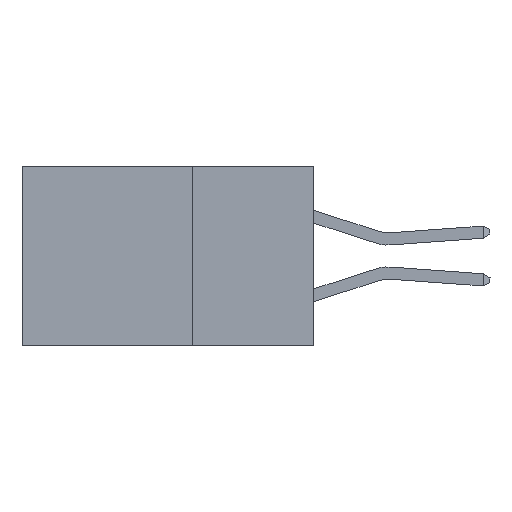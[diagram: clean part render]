
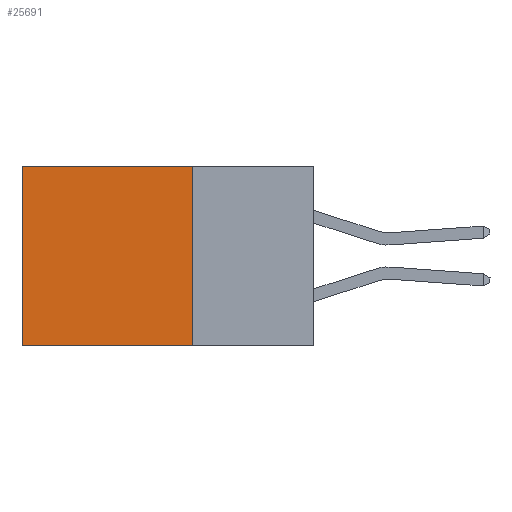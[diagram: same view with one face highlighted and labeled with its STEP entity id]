
A CAD part, left-side view. The second image highlights one B-rep face of the part: STEP entity #25691.
In plain terms, the highlighted planar face has unit normal (-1, 0, 0).
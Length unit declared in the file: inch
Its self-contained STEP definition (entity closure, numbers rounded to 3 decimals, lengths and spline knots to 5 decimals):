
#349 = ORIENTED_EDGE ( 'NONE', *, *, #8918, .F. ) ;
#813 = ORIENTED_EDGE ( 'NONE', *, *, #2365, .F. ) ;
#841 = DIRECTION ( 'NONE',  ( 0., 1., 0. ) ) ;
#2365 = EDGE_CURVE ( 'NONE', #13467, #4650, #9687, .T. ) ;
#3313 = VERTEX_POINT ( 'NONE', #12377 ) ;
#3667 = DIRECTION ( 'NONE',  ( 0., 0., -1. ) ) ;
#4650 = VERTEX_POINT ( 'NONE', #18858 ) ;
#4749 = EDGE_CURVE ( 'NONE', #22105, #4650, #6490, .T. ) ;
#6490 = LINE ( 'NONE', #26032, #29679 ) ;
#8918 = EDGE_CURVE ( 'NONE', #3313, #13467, #23501, .T. ) ;
#9687 = LINE ( 'NONE', #26998, #11532 ) ;
#10871 = CARTESIAN_POINT ( 'NONE',  ( 0.2875, 0.25, 0. ) ) ;
#11532 = VECTOR ( 'NONE', #841, 39.37008 ) ;
#11854 = ORIENTED_EDGE ( 'NONE', *, *, #22484, .T. ) ;
#12377 = CARTESIAN_POINT ( 'NONE',  ( 0.2875, 0.25, 0. ) ) ;
#13467 = VERTEX_POINT ( 'NONE', #18179 ) ;
#15253 = VECTOR ( 'NONE', #17674, 39.37008 ) ;
#15743 = DIRECTION ( 'NONE',  ( 1., 0., 0. ) ) ;
#16172 = EDGE_LOOP ( 'NONE', ( #24055, #813, #349, #11854 ) ) ;
#16554 = AXIS2_PLACEMENT_3D ( 'NONE', #29913, #15743, #3667 ) ;
#17440 = LINE ( 'NONE', #17460, #15253 ) ;
#17460 = CARTESIAN_POINT ( 'NONE',  ( 0.2875, 0.25, 0. ) ) ;
#17674 = DIRECTION ( 'NONE',  ( 0., 1., 0. ) ) ;
#18179 = CARTESIAN_POINT ( 'NONE',  ( 0.2875, 0.25, -0.37 ) ) ;
#18858 = CARTESIAN_POINT ( 'NONE',  ( 0.2875, 0.6, -0.37 ) ) ;
#20506 = CARTESIAN_POINT ( 'NONE',  ( 0.2875, 0.6, 0. ) ) ;
#21051 = DIRECTION ( 'NONE',  ( 0., 0., -1. ) ) ;
#22105 = VERTEX_POINT ( 'NONE', #20506 ) ;
#22484 = EDGE_CURVE ( 'NONE', #3313, #22105, #17440, .T. ) ;
#23501 = LINE ( 'NONE', #10871, #26126 ) ;
#24055 = ORIENTED_EDGE ( 'NONE', *, *, #4749, .T. ) ;
#25049 = DIRECTION ( 'NONE',  ( 0., 0., -1. ) ) ;
#25691 = ADVANCED_FACE ( 'NONE', ( #28789 ), #29593, .F. ) ;
#26032 = CARTESIAN_POINT ( 'NONE',  ( 0.2875, 0.6, 0. ) ) ;
#26126 = VECTOR ( 'NONE', #25049, 39.37008 ) ;
#26998 = CARTESIAN_POINT ( 'NONE',  ( 0.2875, 0.25, -0.37 ) ) ;
#28789 = FACE_OUTER_BOUND ( 'NONE', #16172, .T. ) ;
#29593 = PLANE ( 'NONE',  #16554 ) ;
#29679 = VECTOR ( 'NONE', #21051, 39.37008 ) ;
#29913 = CARTESIAN_POINT ( 'NONE',  ( 0.2875, 0.25, 0. ) ) ;
